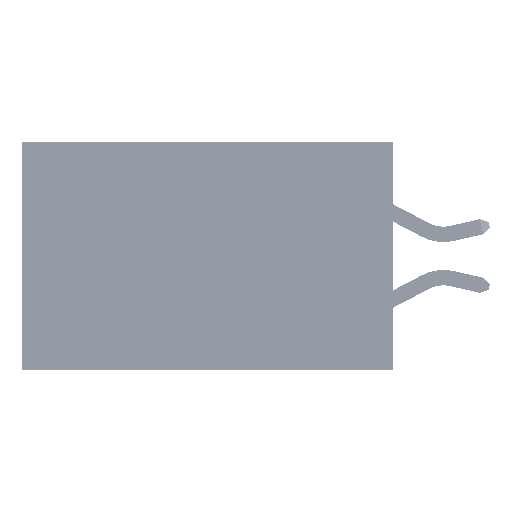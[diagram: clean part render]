
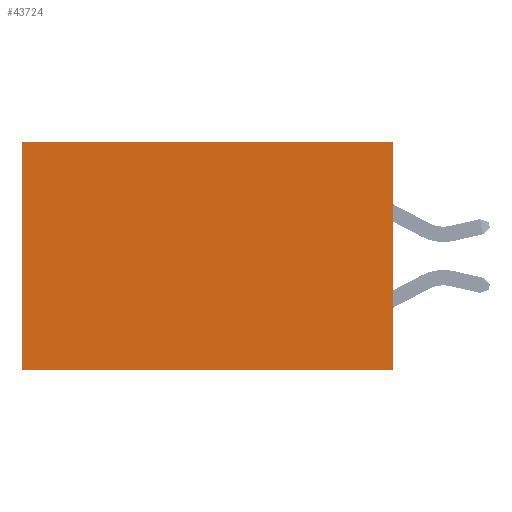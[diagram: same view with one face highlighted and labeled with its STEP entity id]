
A CAD part, left-side view. The second image highlights one B-rep face of the part: STEP entity #43724.
In plain terms, the highlighted planar face has unit normal (-1, 0, 0).
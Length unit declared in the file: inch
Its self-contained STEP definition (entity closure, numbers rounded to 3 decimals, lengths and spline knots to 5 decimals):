
#1894 = LINE ( 'NONE', #37671, #12411 ) ;
#2204 = DIRECTION ( 'NONE',  ( 0., 0., -1. ) ) ;
#2983 = ORIENTED_EDGE ( 'NONE', *, *, #40322, .T. ) ;
#3004 = VECTOR ( 'NONE', #28980, 39.37008 ) ;
#3517 = LINE ( 'NONE', #25707, #3004 ) ;
#5926 = DIRECTION ( 'NONE',  ( 0., 1., 0. ) ) ;
#6798 = FACE_OUTER_BOUND ( 'NONE', #22681, .T. ) ;
#6996 = EDGE_CURVE ( 'NONE', #36305, #23373, #41400, .T. ) ;
#7903 = VECTOR ( 'NONE', #8781, 39.37008 ) ;
#8128 = ORIENTED_EDGE ( 'NONE', *, *, #18516, .T. ) ;
#8720 = AXIS2_PLACEMENT_3D ( 'NONE', #30561, #41912, #2204 ) ;
#8781 = DIRECTION ( 'NONE',  ( 0., 0., -1. ) ) ;
#12411 = VECTOR ( 'NONE', #38003, 39.37008 ) ;
#13528 = CARTESIAN_POINT ( 'NONE',  ( 0.2875, 0., 0. ) ) ;
#16115 = ORIENTED_EDGE ( 'NONE', *, *, #18087, .F. ) ;
#17386 = CARTESIAN_POINT ( 'NONE',  ( 0.2875, 0.6, 0. ) ) ;
#18087 = EDGE_CURVE ( 'NONE', #32262, #36305, #1894, .T. ) ;
#18516 = EDGE_CURVE ( 'NONE', #37427, #23373, #22901, .T. ) ;
#21453 = CARTESIAN_POINT ( 'NONE',  ( 0.2875, 0., -0.37 ) ) ;
#22681 = EDGE_LOOP ( 'NONE', ( #8128, #45073, #16115, #2983 ) ) ;
#22901 = LINE ( 'NONE', #26766, #7903 ) ;
#23373 = VERTEX_POINT ( 'NONE', #28529 ) ;
#25707 = CARTESIAN_POINT ( 'NONE',  ( 0.2875, 0., 0. ) ) ;
#26766 = CARTESIAN_POINT ( 'NONE',  ( 0.2875, 0.6, 0. ) ) ;
#27623 = CARTESIAN_POINT ( 'NONE',  ( 0.2875, 0., -0.37 ) ) ;
#28043 = VECTOR ( 'NONE', #5926, 39.37008 ) ;
#28529 = CARTESIAN_POINT ( 'NONE',  ( 0.2875, 0.6, -0.37 ) ) ;
#28980 = DIRECTION ( 'NONE',  ( 0., 1., 0. ) ) ;
#30561 = CARTESIAN_POINT ( 'NONE',  ( 0.2875, 0., 0. ) ) ;
#32262 = VERTEX_POINT ( 'NONE', #13528 ) ;
#36305 = VERTEX_POINT ( 'NONE', #21453 ) ;
#37427 = VERTEX_POINT ( 'NONE', #17386 ) ;
#37671 = CARTESIAN_POINT ( 'NONE',  ( 0.2875, 0., 0. ) ) ;
#38003 = DIRECTION ( 'NONE',  ( 0., 0., -1. ) ) ;
#40322 = EDGE_CURVE ( 'NONE', #32262, #37427, #3517, .T. ) ;
#41400 = LINE ( 'NONE', #27623, #28043 ) ;
#41912 = DIRECTION ( 'NONE',  ( 1., 0., 0. ) ) ;
#43724 = ADVANCED_FACE ( 'NONE', ( #6798 ), #44980, .F. ) ;
#44980 = PLANE ( 'NONE',  #8720 ) ;
#45073 = ORIENTED_EDGE ( 'NONE', *, *, #6996, .F. ) ;
